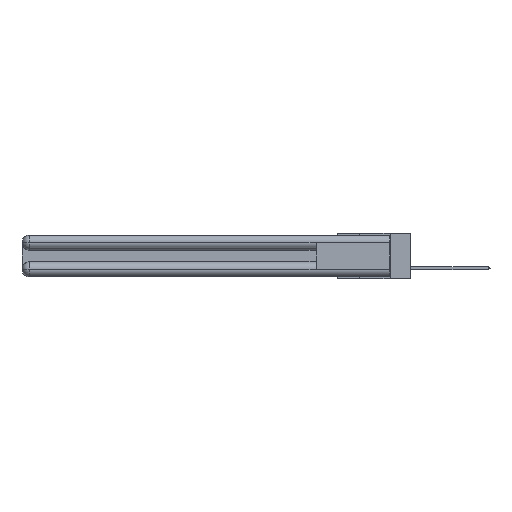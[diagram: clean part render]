
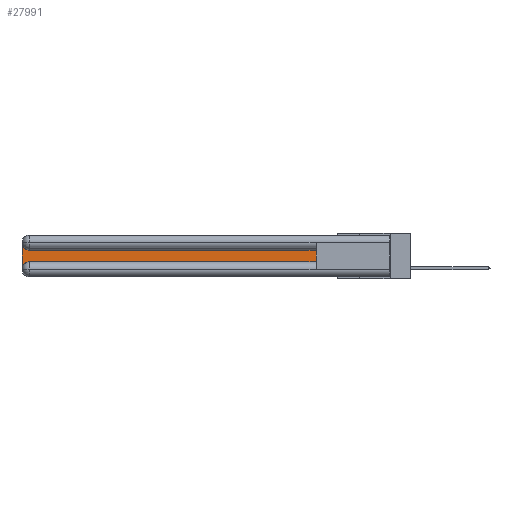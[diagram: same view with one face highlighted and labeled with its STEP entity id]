
A CAD part, left-side view. The second image highlights one B-rep face of the part: STEP entity #27991.
In plain terms, the highlighted planar face has unit normal (-1, 0, 0).
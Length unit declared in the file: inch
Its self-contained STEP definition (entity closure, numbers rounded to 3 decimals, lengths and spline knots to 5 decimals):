
#113 = DIRECTION ( 'NONE',  ( 0., 0., -1. ) ) ;
#1526 = CARTESIAN_POINT ( 'NONE',  ( 0.075, 3., -0.0625 ) ) ;
#1558 = EDGE_CURVE ( 'NONE', #3540, #3334, #16792, .T. ) ;
#2514 = ORIENTED_EDGE ( 'NONE', *, *, #14153, .T. ) ;
#3264 = VECTOR ( 'NONE', #113, 39.37008 ) ;
#3334 = VERTEX_POINT ( 'NONE', #16599 ) ;
#3341 = EDGE_CURVE ( 'NONE', #3334, #16953, #14632, .T. ) ;
#3466 = CARTESIAN_POINT ( 'NONE',  ( 0.075, 2.94, -0.0625 ) ) ;
#3540 = VERTEX_POINT ( 'NONE', #6827 ) ;
#4251 = CARTESIAN_POINT ( 'NONE',  ( 0.075, 3., -0.2175 ) ) ;
#4422 = AXIS2_PLACEMENT_3D ( 'NONE', #3466, #18818, #10085 ) ;
#4602 = LINE ( 'NONE', #5745, #17656 ) ;
#5097 = VECTOR ( 'NONE', #21015, 39.37008 ) ;
#5745 = CARTESIAN_POINT ( 'NONE',  ( 0.075, 0.6, -0.2175 ) ) ;
#6187 = EDGE_CURVE ( 'NONE', #28141, #3540, #21427, .T. ) ;
#6827 = CARTESIAN_POINT ( 'NONE',  ( 0.075, 0.6, -0.1225 ) ) ;
#8165 = CARTESIAN_POINT ( 'NONE',  ( 0.075, 2.94, -0.2175 ) ) ;
#9041 = VECTOR ( 'NONE', #19101, 39.37008 ) ;
#10085 = DIRECTION ( 'NONE',  ( 0., 0., -1. ) ) ;
#10545 = CARTESIAN_POINT ( 'NONE',  ( 0.075, 0.6, -0.2175 ) ) ;
#10578 = PLANE ( 'NONE',  #12651 ) ;
#11168 = CIRCLE ( 'NONE', #20807, 0.06 ) ;
#12122 = EDGE_LOOP ( 'NONE', ( #15045, #25526, #22709, #24862, #2514, #28341 ) ) ;
#12375 = DIRECTION ( 'NONE',  ( 0., -1., 0. ) ) ;
#12651 = AXIS2_PLACEMENT_3D ( 'NONE', #14608, #23478, #16907 ) ;
#13892 = CARTESIAN_POINT ( 'NONE',  ( 0.075, 0.6, -0.1225 ) ) ;
#14153 = EDGE_CURVE ( 'NONE', #16954, #28141, #4602, .T. ) ;
#14272 = CARTESIAN_POINT ( 'NONE',  ( 0.075, 3., -0.2775 ) ) ;
#14608 = CARTESIAN_POINT ( 'NONE',  ( 0.075, 3., -0.1225 ) ) ;
#14632 = CIRCLE ( 'NONE', #4422, 0.06 ) ;
#15045 = ORIENTED_EDGE ( 'NONE', *, *, #1558, .T. ) ;
#16599 = CARTESIAN_POINT ( 'NONE',  ( 0.075, 2.94, -0.1225 ) ) ;
#16792 = LINE ( 'NONE', #13892, #5097 ) ;
#16907 = DIRECTION ( 'NONE',  ( 0., 0., -1. ) ) ;
#16953 = VERTEX_POINT ( 'NONE', #1526 ) ;
#16954 = VERTEX_POINT ( 'NONE', #8165 ) ;
#17403 = CARTESIAN_POINT ( 'NONE',  ( 0.075, 2.94, -0.2775 ) ) ;
#17656 = VECTOR ( 'NONE', #12375, 39.37008 ) ;
#17932 = FACE_OUTER_BOUND ( 'NONE', #12122, .T. ) ;
#18464 = EDGE_CURVE ( 'NONE', #21486, #16954, #11168, .T. ) ;
#18470 = EDGE_CURVE ( 'NONE', #16953, #21486, #23572, .T. ) ;
#18818 = DIRECTION ( 'NONE',  ( 1., 0., 0. ) ) ;
#19101 = DIRECTION ( 'NONE',  ( 0., 0., 1. ) ) ;
#19104 = CARTESIAN_POINT ( 'NONE',  ( 0.075, 0.6, -0.2175 ) ) ;
#19540 = DIRECTION ( 'NONE',  ( 0., 0., -1. ) ) ;
#20807 = AXIS2_PLACEMENT_3D ( 'NONE', #17403, #22049, #19540 ) ;
#21015 = DIRECTION ( 'NONE',  ( 0., 1., 0. ) ) ;
#21427 = LINE ( 'NONE', #10545, #9041 ) ;
#21486 = VERTEX_POINT ( 'NONE', #14272 ) ;
#22049 = DIRECTION ( 'NONE',  ( 1., 0., 0. ) ) ;
#22709 = ORIENTED_EDGE ( 'NONE', *, *, #18470, .T. ) ;
#23478 = DIRECTION ( 'NONE',  ( 1., 0., 0. ) ) ;
#23572 = LINE ( 'NONE', #4251, #3264 ) ;
#24862 = ORIENTED_EDGE ( 'NONE', *, *, #18464, .T. ) ;
#25526 = ORIENTED_EDGE ( 'NONE', *, *, #3341, .T. ) ;
#27991 = ADVANCED_FACE ( 'NONE', ( #17932 ), #10578, .F. ) ;
#28141 = VERTEX_POINT ( 'NONE', #19104 ) ;
#28341 = ORIENTED_EDGE ( 'NONE', *, *, #6187, .T. ) ;
